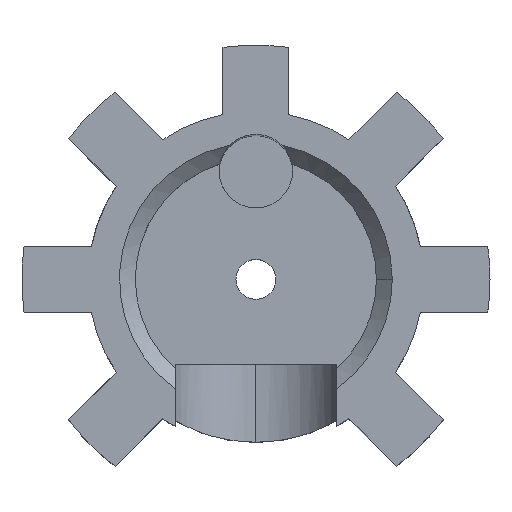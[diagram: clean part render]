
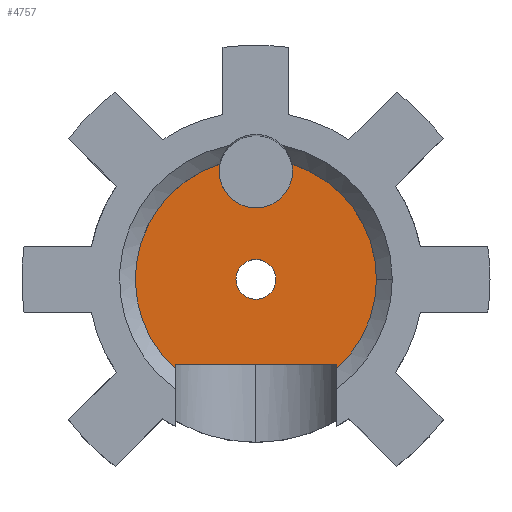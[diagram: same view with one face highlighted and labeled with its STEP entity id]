
A CAD part, top view. The second image highlights one B-rep face of the part: STEP entity #4757.
In plain terms, the highlighted planar face has unit normal (0, 0, 1).
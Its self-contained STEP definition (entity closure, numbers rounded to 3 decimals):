
#29 = EDGE_LOOP ( 'NONE', ( #294, #1185 ) ) ;
#53 = CARTESIAN_POINT ( 'NONE',  ( -1.447, 4.617, -3.175 ) ) ;
#294 = ORIENTED_EDGE ( 'NONE', *, *, #1876, .T. ) ;
#466 = EDGE_CURVE ( 'NONE', #3471, #3248, #826, .T. ) ;
#501 = CIRCLE ( 'NONE', #1471, 1.473 ) ;
#540 = AXIS2_PLACEMENT_3D ( 'NONE', #5403, #5387, #5018 ) ;
#554 = CARTESIAN_POINT ( 'NONE',  ( 4.839, 0., -3.175 ) ) ;
#606 = DIRECTION ( 'NONE',  ( 1., 0., 0. ) ) ;
#626 = VECTOR ( 'NONE', #4215, 1000. ) ;
#823 = VERTEX_POINT ( 'NONE', #2565 ) ;
#826 = CIRCLE ( 'NONE', #4365, 1.473 ) ;
#881 = AXIS2_PLACEMENT_3D ( 'NONE', #3798, #3732, #3716 ) ;
#901 = EDGE_CURVE ( 'NONE', #5231, #2781, #5190, .T. ) ;
#960 = VECTOR ( 'NONE', #2814, 1000. ) ;
#970 = EDGE_CURVE ( 'NONE', #5318, #823, #5140, .T. ) ;
#1005 = EDGE_CURVE ( 'NONE', #2812, #2453, #1804, .T. ) ;
#1018 = CARTESIAN_POINT ( 'NONE',  ( 3.239, -3.429, -3.175 ) ) ;
#1081 = CARTESIAN_POINT ( 'NONE',  ( -3.239, 0., -3.175 ) ) ;
#1159 = EDGE_CURVE ( 'NONE', #5269, #2812, #4387, .T. ) ;
#1180 = DIRECTION ( 'NONE',  ( 0., 0., -1. ) ) ;
#1181 = VERTEX_POINT ( 'NONE', #5114 ) ;
#1185 = ORIENTED_EDGE ( 'NONE', *, *, #3702, .T. ) ;
#1235 = CARTESIAN_POINT ( 'NONE',  ( 0., 0., -3.175 ) ) ;
#1311 = ORIENTED_EDGE ( 'NONE', *, *, #3586, .T. ) ;
#1368 = VERTEX_POINT ( 'NONE', #2504 ) ;
#1381 = ORIENTED_EDGE ( 'NONE', *, *, #970, .T. ) ;
#1395 = CIRCLE ( 'NONE', #3518, 0.8 ) ;
#1422 = CARTESIAN_POINT ( 'NONE',  ( -3.239, -3.595, -3.175 ) ) ;
#1470 = PLANE ( 'NONE',  #2717 ) ;
#1471 = AXIS2_PLACEMENT_3D ( 'NONE', #2407, #5305, #2848 ) ;
#1523 = ORIENTED_EDGE ( 'NONE', *, *, #5010, .T. ) ;
#1541 = DIRECTION ( 'NONE',  ( 0., 0., 1. ) ) ;
#1687 = DIRECTION ( 'NONE',  ( 1., 0., 0. ) ) ;
#1781 = AXIS2_PLACEMENT_3D ( 'NONE', #4111, #1541, #4522 ) ;
#1804 = LINE ( 'NONE', #4139, #626 ) ;
#1822 = FACE_OUTER_BOUND ( 'NONE', #4347, .T. ) ;
#1876 = EDGE_CURVE ( 'NONE', #1368, #1181, #1395, .T. ) ;
#1890 = ORIENTED_EDGE ( 'NONE', *, *, #466, .T. ) ;
#1896 = CIRCLE ( 'NONE', #4640, 0.8 ) ;
#1934 = DIRECTION ( 'NONE',  ( 0., 0., 1. ) ) ;
#2046 = ORIENTED_EDGE ( 'NONE', *, *, #4907, .T. ) ;
#2060 = CARTESIAN_POINT ( 'NONE',  ( 0., 4.341, -3.175 ) ) ;
#2187 = DIRECTION ( 'NONE',  ( 0., 0., -1. ) ) ;
#2342 = ORIENTED_EDGE ( 'NONE', *, *, #901, .T. ) ;
#2407 = CARTESIAN_POINT ( 'NONE',  ( 0., 4.341, -3.175 ) ) ;
#2422 = ORIENTED_EDGE ( 'NONE', *, *, #4326, .T. ) ;
#2437 = VECTOR ( 'NONE', #4511, 1000. ) ;
#2453 = VERTEX_POINT ( 'NONE', #3373 ) ;
#2465 = DIRECTION ( 'NONE',  ( 1., 0., 0. ) ) ;
#2504 = CARTESIAN_POINT ( 'NONE',  ( 0.8, 0., -3.175 ) ) ;
#2564 = ORIENTED_EDGE ( 'NONE', *, *, #1159, .T. ) ;
#2565 = CARTESIAN_POINT ( 'NONE',  ( 1.447, 4.617, -3.175 ) ) ;
#2717 = AXIS2_PLACEMENT_3D ( 'NONE', #4037, #1934, #4868 ) ;
#2726 = CARTESIAN_POINT ( 'NONE',  ( -3.239, -3.429, -3.175 ) ) ;
#2781 = VERTEX_POINT ( 'NONE', #1422 ) ;
#2783 = CARTESIAN_POINT ( 'NONE',  ( -1.473, 4.341, -3.175 ) ) ;
#2812 = VERTEX_POINT ( 'NONE', #1018 ) ;
#2814 = DIRECTION ( 'NONE',  ( 1., 0., 0. ) ) ;
#2836 = FACE_BOUND ( 'NONE', #29, .T. ) ;
#2848 = DIRECTION ( 'NONE',  ( 1., 0., 0. ) ) ;
#2923 = CARTESIAN_POINT ( 'NONE',  ( 0., 4.341, -3.175 ) ) ;
#3215 = CARTESIAN_POINT ( 'NONE',  ( 0., -3.429, -3.175 ) ) ;
#3248 = VERTEX_POINT ( 'NONE', #2783 ) ;
#3294 = CIRCLE ( 'NONE', #5094, 1.473 ) ;
#3373 = CARTESIAN_POINT ( 'NONE',  ( 3.238, -3.595, -3.175 ) ) ;
#3471 = VERTEX_POINT ( 'NONE', #5113 ) ;
#3518 = AXIS2_PLACEMENT_3D ( 'NONE', #4701, #2187, #5095 ) ;
#3548 = ORIENTED_EDGE ( 'NONE', *, *, #1005, .T. ) ;
#3586 = EDGE_CURVE ( 'NONE', #2453, #5318, #4544, .T. ) ;
#3693 = LINE ( 'NONE', #1081, #2437 ) ;
#3702 = EDGE_CURVE ( 'NONE', #1181, #1368, #1896, .T. ) ;
#3716 = DIRECTION ( 'NONE',  ( 1., 0., 0. ) ) ;
#3732 = DIRECTION ( 'NONE',  ( 0., 0., 1. ) ) ;
#3798 = CARTESIAN_POINT ( 'NONE',  ( 0., 0., -3.175 ) ) ;
#4037 = CARTESIAN_POINT ( 'NONE',  ( 0., 0., -3.175 ) ) ;
#4111 = CARTESIAN_POINT ( 'NONE',  ( 0., 0., -3.175 ) ) ;
#4139 = CARTESIAN_POINT ( 'NONE',  ( 3.239, -7.512, -3.175 ) ) ;
#4215 = DIRECTION ( 'NONE',  ( 0., -1., 0. ) ) ;
#4251 = DIRECTION ( 'NONE',  ( 0., 0., -1. ) ) ;
#4326 = EDGE_CURVE ( 'NONE', #2781, #5269, #3693, .T. ) ;
#4347 = EDGE_LOOP ( 'NONE', ( #1311, #1381, #1523, #1890, #2046, #2342, #2422, #2564, #3548 ) ) ;
#4365 = AXIS2_PLACEMENT_3D ( 'NONE', #2923, #1180, #606 ) ;
#4387 = LINE ( 'NONE', #3215, #960 ) ;
#4511 = DIRECTION ( 'NONE',  ( 0., 1., 0. ) ) ;
#4522 = DIRECTION ( 'NONE',  ( 1., 0., 0. ) ) ;
#4544 = CIRCLE ( 'NONE', #1781, 4.839 ) ;
#4640 = AXIS2_PLACEMENT_3D ( 'NONE', #1235, #4251, #1687 ) ;
#4701 = CARTESIAN_POINT ( 'NONE',  ( 0., 0., -3.175 ) ) ;
#4757 = ADVANCED_FACE ( 'NONE', ( #2836, #1822 ), #1470, .T. ) ;
#4868 = DIRECTION ( 'NONE',  ( 1., 0., 0. ) ) ;
#4907 = EDGE_CURVE ( 'NONE', #3248, #5231, #501, .T. ) ;
#4971 = DIRECTION ( 'NONE',  ( 0., 0., -1. ) ) ;
#5010 = EDGE_CURVE ( 'NONE', #823, #3471, #3294, .T. ) ;
#5018 = DIRECTION ( 'NONE',  ( 1., 0., 0. ) ) ;
#5094 = AXIS2_PLACEMENT_3D ( 'NONE', #2060, #4971, #2465 ) ;
#5095 = DIRECTION ( 'NONE',  ( 1., 0., 0. ) ) ;
#5113 = CARTESIAN_POINT ( 'NONE',  ( 1.473, 4.341, -3.175 ) ) ;
#5114 = CARTESIAN_POINT ( 'NONE',  ( -0.8, 0., -3.175 ) ) ;
#5140 = CIRCLE ( 'NONE', #881, 4.839 ) ;
#5190 = CIRCLE ( 'NONE', #540, 4.839 ) ;
#5231 = VERTEX_POINT ( 'NONE', #53 ) ;
#5269 = VERTEX_POINT ( 'NONE', #2726 ) ;
#5305 = DIRECTION ( 'NONE',  ( 0., 0., -1. ) ) ;
#5318 = VERTEX_POINT ( 'NONE', #554 ) ;
#5387 = DIRECTION ( 'NONE',  ( 0., 0., 1. ) ) ;
#5403 = CARTESIAN_POINT ( 'NONE',  ( 0., 0., -3.175 ) ) ;
